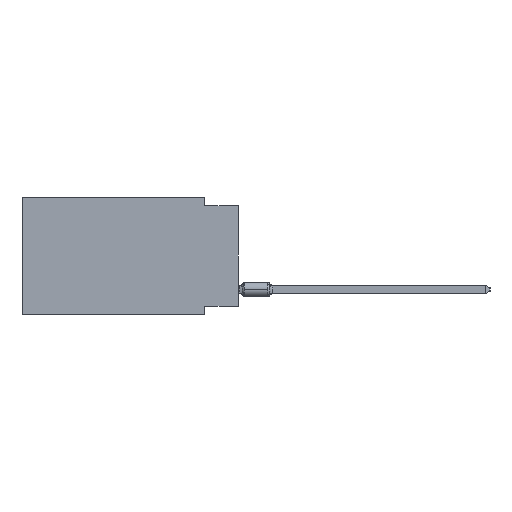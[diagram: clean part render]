
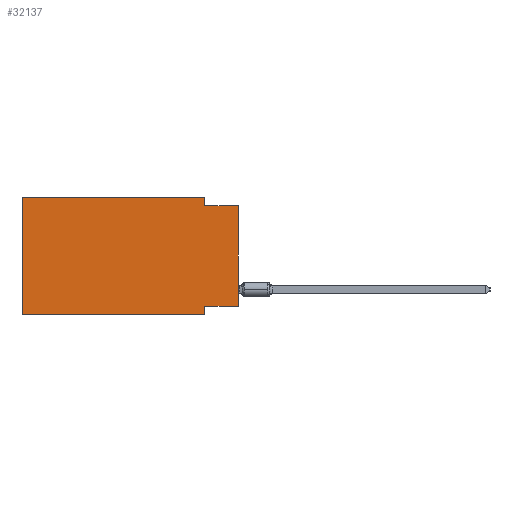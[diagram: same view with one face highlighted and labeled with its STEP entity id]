
A CAD part, left-side view. The second image highlights one B-rep face of the part: STEP entity #32137.
In plain terms, the highlighted planar face has unit normal (-1, 0, 0).
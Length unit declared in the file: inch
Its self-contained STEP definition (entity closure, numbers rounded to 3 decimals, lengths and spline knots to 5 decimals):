
#77 = EDGE_CURVE ( 'NONE', #2478, #10896, #20296, .T. ) ;
#330 = VERTEX_POINT ( 'NONE', #37017 ) ;
#905 = PLANE ( 'NONE',  #27809 ) ;
#1183 = DIRECTION ( 'NONE',  ( 0., -1., 0. ) ) ;
#2088 = VECTOR ( 'NONE', #26167, 39.37008 ) ;
#2478 = VERTEX_POINT ( 'NONE', #25828 ) ;
#2588 = CARTESIAN_POINT ( 'NONE',  ( 0., 0.1, -0.025 ) ) ;
#3410 = CARTESIAN_POINT ( 'NONE',  ( 0., 0.1, -0.35 ) ) ;
#4048 = DIRECTION ( 'NONE',  ( 1., 0., 0. ) ) ;
#4834 = EDGE_CURVE ( 'NONE', #10896, #34823, #35757, .T. ) ;
#4946 = VECTOR ( 'NONE', #38989, 39.37008 ) ;
#7188 = FACE_OUTER_BOUND ( 'NONE', #10291, .T. ) ;
#7271 = ORIENTED_EDGE ( 'NONE', *, *, #29060, .F. ) ;
#8477 = ORIENTED_EDGE ( 'NONE', *, *, #28607, .F. ) ;
#8499 = ORIENTED_EDGE ( 'NONE', *, *, #23000, .F. ) ;
#9231 = VERTEX_POINT ( 'NONE', #18768 ) ;
#9632 = VECTOR ( 'NONE', #1183, 39.37008 ) ;
#9762 = ORIENTED_EDGE ( 'NONE', *, *, #4834, .F. ) ;
#10291 = EDGE_LOOP ( 'NONE', ( #36228, #17633, #8477, #7271, #8499, #38769, #9762, #35203 ) ) ;
#10896 = VERTEX_POINT ( 'NONE', #34374 ) ;
#11241 = CARTESIAN_POINT ( 'NONE',  ( 0., 0.645, 0. ) ) ;
#11973 = CARTESIAN_POINT ( 'NONE',  ( 0., 0.645, -0.35 ) ) ;
#12587 = VECTOR ( 'NONE', #25439, 39.37008 ) ;
#13435 = CARTESIAN_POINT ( 'NONE',  ( 0., 0.645, 0. ) ) ;
#13476 = EDGE_CURVE ( 'NONE', #29522, #330, #34644, .T. ) ;
#14737 = CARTESIAN_POINT ( 'NONE',  ( 0., 0.645, -0.35 ) ) ;
#15297 = EDGE_CURVE ( 'NONE', #2478, #330, #41122, .T. ) ;
#15442 = EDGE_CURVE ( 'NONE', #26606, #34823, #23509, .T. ) ;
#15840 = CARTESIAN_POINT ( 'NONE',  ( 0., 0., -0.025 ) ) ;
#17633 = ORIENTED_EDGE ( 'NONE', *, *, #13476, .F. ) ;
#17845 = VERTEX_POINT ( 'NONE', #37839 ) ;
#18768 = CARTESIAN_POINT ( 'NONE',  ( 0., 0.645, 0. ) ) ;
#20296 = LINE ( 'NONE', #33263, #2088 ) ;
#20476 = VECTOR ( 'NONE', #39646, 39.37008 ) ;
#23000 = EDGE_CURVE ( 'NONE', #26606, #9231, #39759, .T. ) ;
#23126 = VECTOR ( 'NONE', #39704, 39.37008 ) ;
#23509 = LINE ( 'NONE', #14737, #9632 ) ;
#24227 = CARTESIAN_POINT ( 'NONE',  ( 0., 0.1, 0. ) ) ;
#25439 = DIRECTION ( 'NONE',  ( 0., -1., 0. ) ) ;
#25828 = CARTESIAN_POINT ( 'NONE',  ( 0., 0., -0.325 ) ) ;
#26167 = DIRECTION ( 'NONE',  ( 0., 1., 0. ) ) ;
#26270 = VECTOR ( 'NONE', #36409, 39.37008 ) ;
#26606 = VERTEX_POINT ( 'NONE', #11973 ) ;
#27809 = AXIS2_PLACEMENT_3D ( 'NONE', #13435, #4048, #37033 ) ;
#28607 = EDGE_CURVE ( 'NONE', #17845, #29522, #33635, .T. ) ;
#29060 = EDGE_CURVE ( 'NONE', #9231, #17845, #39242, .T. ) ;
#29522 = VERTEX_POINT ( 'NONE', #2588 ) ;
#31706 = CARTESIAN_POINT ( 'NONE',  ( 0., 0., 0. ) ) ;
#32137 = ADVANCED_FACE ( 'NONE', ( #7188 ), #905, .F. ) ;
#33263 = CARTESIAN_POINT ( 'NONE',  ( 0., 0., -0.325 ) ) ;
#33283 = CARTESIAN_POINT ( 'NONE',  ( 0., 0.645, 0. ) ) ;
#33635 = LINE ( 'NONE', #24227, #23126 ) ;
#34374 = CARTESIAN_POINT ( 'NONE',  ( 0., 0.1, -0.325 ) ) ;
#34644 = LINE ( 'NONE', #15840, #12587 ) ;
#34688 = CARTESIAN_POINT ( 'NONE',  ( 0., 0.1, -0.35 ) ) ;
#34823 = VERTEX_POINT ( 'NONE', #34688 ) ;
#35203 = ORIENTED_EDGE ( 'NONE', *, *, #77, .F. ) ;
#35367 = DIRECTION ( 'NONE',  ( 0., 0., -1. ) ) ;
#35757 = LINE ( 'NONE', #3410, #37781 ) ;
#36228 = ORIENTED_EDGE ( 'NONE', *, *, #15297, .T. ) ;
#36409 = DIRECTION ( 'NONE',  ( 0., 0., 1. ) ) ;
#37017 = CARTESIAN_POINT ( 'NONE',  ( 0., 0., -0.025 ) ) ;
#37033 = DIRECTION ( 'NONE',  ( 0., 0., -1. ) ) ;
#37781 = VECTOR ( 'NONE', #35367, 39.37008 ) ;
#37839 = CARTESIAN_POINT ( 'NONE',  ( 0., 0.1, 0. ) ) ;
#38769 = ORIENTED_EDGE ( 'NONE', *, *, #15442, .T. ) ;
#38989 = DIRECTION ( 'NONE',  ( 0., 0., 1. ) ) ;
#39242 = LINE ( 'NONE', #11241, #20476 ) ;
#39646 = DIRECTION ( 'NONE',  ( 0., -1., 0. ) ) ;
#39704 = DIRECTION ( 'NONE',  ( 0., 0., -1. ) ) ;
#39759 = LINE ( 'NONE', #33283, #26270 ) ;
#41122 = LINE ( 'NONE', #31706, #4946 ) ;
